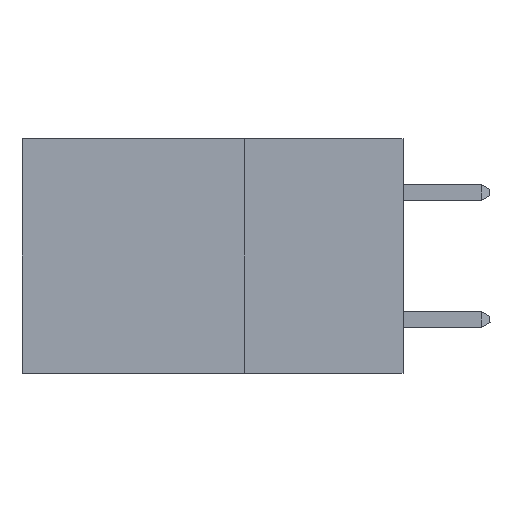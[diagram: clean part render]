
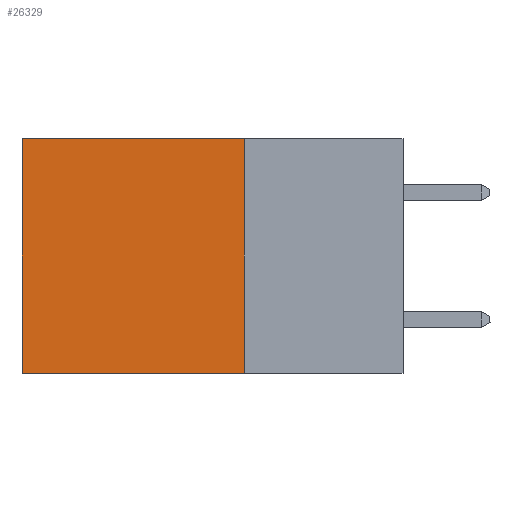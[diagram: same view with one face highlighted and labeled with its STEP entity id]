
A CAD part, left-side view. The second image highlights one B-rep face of the part: STEP entity #26329.
In plain terms, the highlighted planar face has unit normal (-1, 0, 0).
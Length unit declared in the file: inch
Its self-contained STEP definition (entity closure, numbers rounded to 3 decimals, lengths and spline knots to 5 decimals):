
#765 = VERTEX_POINT ( 'NONE', #4029 ) ;
#1144 = EDGE_CURVE ( 'NONE', #20624, #765, #15518, .T. ) ;
#1305 = DIRECTION ( 'NONE',  ( 0., 0., -1. ) ) ;
#1482 = CARTESIAN_POINT ( 'NONE',  ( 0.2875, 0.6, 0. ) ) ;
#2442 = CARTESIAN_POINT ( 'NONE',  ( 0.2875, 0.25, 0. ) ) ;
#4029 = CARTESIAN_POINT ( 'NONE',  ( 0.2875, 0.6, 0. ) ) ;
#4723 = DIRECTION ( 'NONE',  ( 0., 1., 0. ) ) ;
#5617 = EDGE_LOOP ( 'NONE', ( #13858, #7837, #24953, #20950 ) ) ;
#5672 = DIRECTION ( 'NONE',  ( 1., 0., 0. ) ) ;
#6141 = LINE ( 'NONE', #1482, #16785 ) ;
#6198 = EDGE_CURVE ( 'NONE', #8953, #7286, #9713, .T. ) ;
#6305 = CARTESIAN_POINT ( 'NONE',  ( 0.2875, 0.6, -0.37 ) ) ;
#7286 = VERTEX_POINT ( 'NONE', #6305 ) ;
#7288 = VECTOR ( 'NONE', #20239, 39.37008 ) ;
#7762 = PLANE ( 'NONE',  #22684 ) ;
#7837 = ORIENTED_EDGE ( 'NONE', *, *, #6198, .F. ) ;
#8530 = EDGE_CURVE ( 'NONE', #20624, #8953, #23090, .T. ) ;
#8953 = VERTEX_POINT ( 'NONE', #27376 ) ;
#9713 = LINE ( 'NONE', #11116, #22037 ) ;
#9944 = FACE_OUTER_BOUND ( 'NONE', #5617, .T. ) ;
#10073 = VECTOR ( 'NONE', #15067, 39.37008 ) ;
#10839 = CARTESIAN_POINT ( 'NONE',  ( 0.2875, 0.25, 0. ) ) ;
#10922 = CARTESIAN_POINT ( 'NONE',  ( 0.2875, 0.25, 0. ) ) ;
#11116 = CARTESIAN_POINT ( 'NONE',  ( 0.2875, 0.25, -0.37 ) ) ;
#13858 = ORIENTED_EDGE ( 'NONE', *, *, #15758, .T. ) ;
#15067 = DIRECTION ( 'NONE',  ( 0., 0., -1. ) ) ;
#15518 = LINE ( 'NONE', #26532, #7288 ) ;
#15758 = EDGE_CURVE ( 'NONE', #765, #7286, #6141, .T. ) ;
#16785 = VECTOR ( 'NONE', #27598, 39.37008 ) ;
#20239 = DIRECTION ( 'NONE',  ( 0., 1., 0. ) ) ;
#20624 = VERTEX_POINT ( 'NONE', #10922 ) ;
#20950 = ORIENTED_EDGE ( 'NONE', *, *, #1144, .T. ) ;
#22037 = VECTOR ( 'NONE', #4723, 39.37008 ) ;
#22684 = AXIS2_PLACEMENT_3D ( 'NONE', #2442, #5672, #1305 ) ;
#23090 = LINE ( 'NONE', #10839, #10073 ) ;
#24953 = ORIENTED_EDGE ( 'NONE', *, *, #8530, .F. ) ;
#26329 = ADVANCED_FACE ( 'NONE', ( #9944 ), #7762, .F. ) ;
#26532 = CARTESIAN_POINT ( 'NONE',  ( 0.2875, 0.25, 0. ) ) ;
#27376 = CARTESIAN_POINT ( 'NONE',  ( 0.2875, 0.25, -0.37 ) ) ;
#27598 = DIRECTION ( 'NONE',  ( 0., 0., -1. ) ) ;
